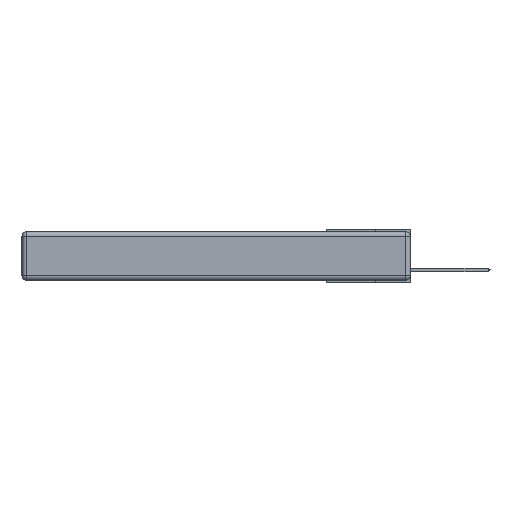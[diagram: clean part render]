
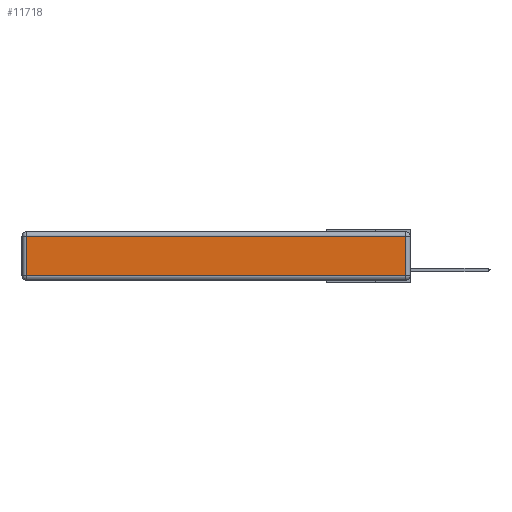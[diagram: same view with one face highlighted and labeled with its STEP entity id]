
A CAD part, left-side view. The second image highlights one B-rep face of the part: STEP entity #11718.
In plain terms, the highlighted planar face has unit normal (-1, 0, 0).
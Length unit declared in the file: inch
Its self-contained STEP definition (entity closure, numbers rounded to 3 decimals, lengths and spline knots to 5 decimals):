
#134 = CARTESIAN_POINT ( 'NONE',  ( 0., 2.72, -0.313 ) ) ;
#3445 = PLANE ( 'NONE',  #4516 ) ;
#4516 = AXIS2_PLACEMENT_3D ( 'NONE', #29884, #14283, #11500 ) ;
#4830 = LINE ( 'NONE', #19029, #17396 ) ;
#4861 = CARTESIAN_POINT ( 'NONE',  ( 0., 2.72, -0.03 ) ) ;
#5849 = CARTESIAN_POINT ( 'NONE',  ( 0., 0.03, -0.313 ) ) ;
#7187 = CARTESIAN_POINT ( 'NONE',  ( 0., 2.72, -0.343 ) ) ;
#8380 = EDGE_CURVE ( 'NONE', #13784, #29650, #20971, .T. ) ;
#8753 = LINE ( 'NONE', #32500, #26766 ) ;
#11371 = VERTEX_POINT ( 'NONE', #4861 ) ;
#11500 = DIRECTION ( 'NONE',  ( 0., 0., 1. ) ) ;
#11718 = ADVANCED_FACE ( 'NONE', ( #16428 ), #3445, .T. ) ;
#12788 = LINE ( 'NONE', #7187, #28726 ) ;
#13053 = VERTEX_POINT ( 'NONE', #134 ) ;
#13409 = VECTOR ( 'NONE', #21272, 39.37008 ) ;
#13784 = VERTEX_POINT ( 'NONE', #5849 ) ;
#14283 = DIRECTION ( 'NONE',  ( -1., 0., 0. ) ) ;
#14942 = EDGE_CURVE ( 'NONE', #13053, #13784, #4830, .T. ) ;
#16428 = FACE_OUTER_BOUND ( 'NONE', #32547, .T. ) ;
#17396 = VECTOR ( 'NONE', #21352, 39.37008 ) ;
#17606 = ORIENTED_EDGE ( 'NONE', *, *, #8380, .T. ) ;
#19029 = CARTESIAN_POINT ( 'NONE',  ( 0., 0., -0.313 ) ) ;
#20971 = LINE ( 'NONE', #24090, #13409 ) ;
#21272 = DIRECTION ( 'NONE',  ( 0., 0., 1. ) ) ;
#21345 = ORIENTED_EDGE ( 'NONE', *, *, #14942, .T. ) ;
#21352 = DIRECTION ( 'NONE',  ( 0., -1., 0. ) ) ;
#22606 = EDGE_CURVE ( 'NONE', #11371, #13053, #12788, .T. ) ;
#24090 = CARTESIAN_POINT ( 'NONE',  ( 0., 0.03, -0.343 ) ) ;
#26766 = VECTOR ( 'NONE', #29364, 39.37008 ) ;
#26920 = EDGE_CURVE ( 'NONE', #29650, #11371, #8753, .T. ) ;
#28726 = VECTOR ( 'NONE', #33932, 39.37008 ) ;
#29364 = DIRECTION ( 'NONE',  ( 0., 1., 0. ) ) ;
#29650 = VERTEX_POINT ( 'NONE', #30946 ) ;
#29884 = CARTESIAN_POINT ( 'NONE',  ( 0., 0., -0.343 ) ) ;
#29965 = ORIENTED_EDGE ( 'NONE', *, *, #26920, .T. ) ;
#29982 = ORIENTED_EDGE ( 'NONE', *, *, #22606, .T. ) ;
#30946 = CARTESIAN_POINT ( 'NONE',  ( 0., 0.03, -0.03 ) ) ;
#32500 = CARTESIAN_POINT ( 'NONE',  ( 0., 2.75, -0.03 ) ) ;
#32547 = EDGE_LOOP ( 'NONE', ( #21345, #17606, #29965, #29982 ) ) ;
#33932 = DIRECTION ( 'NONE',  ( 0., 0., -1. ) ) ;
